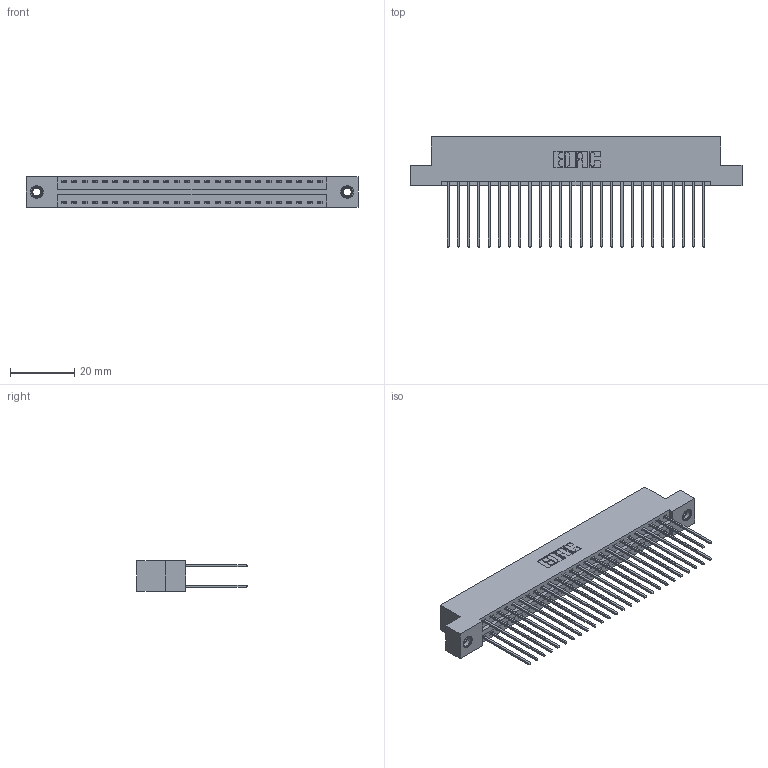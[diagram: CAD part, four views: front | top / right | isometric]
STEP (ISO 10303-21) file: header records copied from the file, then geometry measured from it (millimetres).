
FILE_DESCRIPTION (( 'STEP AP203' ), '1' );
FILE_NAME ('396-052-541-207.STEP', '2018-09-08T06:26:59', ( '' ), ( '' ), 'SwSTEP 2.0', 'SolidWorks 2016', '' );
FILE_SCHEMA (( 'CONFIG_CONTROL_DESIGN' ));
Length unit declared in the file: inch
Products named in the file (4): 345-292-001_345-293-141; 345-250-001_345-250-005-103; 396-052-541-207; 346 Part_Flush Mounting Lugs - 0.156 Dia-TI
Assembly tree (55 placements, depth 2):
  396-052-541-207
    346 Part_Flush Mounting Lugs - 0.156 Dia-TI
    345-292-001_345-293-141  x52
    345-250-001_345-250-005-103  x2
Bounding box: 103.12 x 34.29 x 9.4 mm (x, y, z)
Volume: 10216.4 mm3; surface area: 15256.2 mm2
Topology: 55 solids, 55 shells, 2886 faces, 8525 edges, 5606 vertices
Faces by surface type: plane 1928, cylinder 942, cone 12, torus 4
Entity records: 20326 total; most frequent: CARTESIAN_POINT 3355, ORIENTED_EDGE 3282, DIRECTION 3035, EDGE_CURVE 1641, LINE 1385, VECTOR 1385, VERTEX_POINT 1088, AXIS2_PLACEMENT_3D 825
